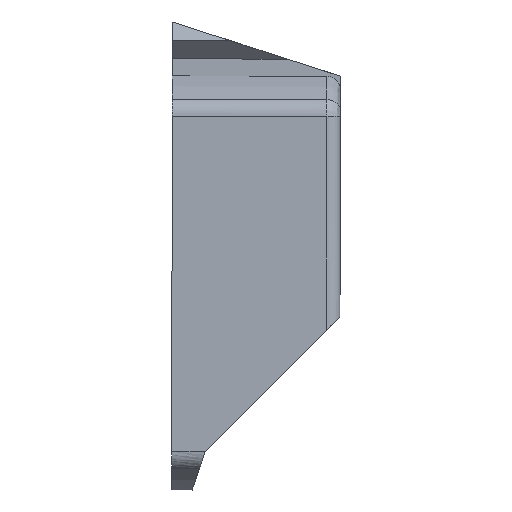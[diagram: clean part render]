
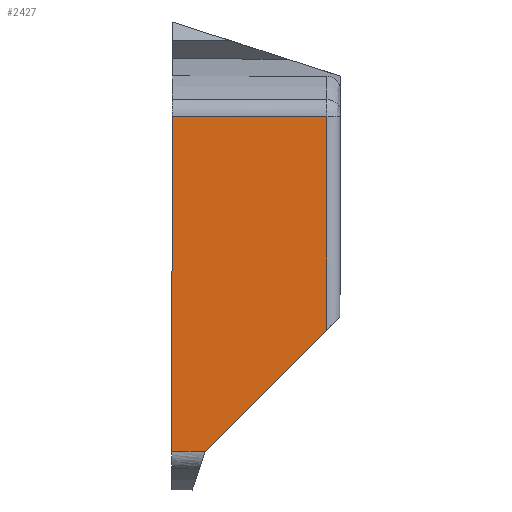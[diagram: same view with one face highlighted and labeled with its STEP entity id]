
A CAD part, front view. The second image highlights one B-rep face of the part: STEP entity #2427.
In plain terms, the highlighted planar face has unit normal (0, -1, 0).
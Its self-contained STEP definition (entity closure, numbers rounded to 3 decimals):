
#143=PLANE('',#2512);
#271=FACE_OUTER_BOUND('',#417,.T.);
#417=EDGE_LOOP('',(#2188,#2189,#2190,#2191,#2192,#2193));
#497=LINE('',#4180,#661);
#512=LINE('',#4357,#676);
#544=LINE('',#4589,#708);
#556=LINE('',#4790,#720);
#582=LINE('',#4938,#746);
#583=LINE('',#4939,#747);
#661=VECTOR('',#2600,10.);
#676=VECTOR('',#2637,10.);
#708=VECTOR('',#2695,10.);
#720=VECTOR('',#2737,10.);
#746=VECTOR('',#2803,10.);
#747=VECTOR('',#2804,10.);
#1038=VERTEX_POINT('',#4176);
#1040=VERTEX_POINT('',#4179);
#1071=VERTEX_POINT('',#4354);
#1072=VERTEX_POINT('',#4356);
#1112=VERTEX_POINT('',#4578);
#1133=VERTEX_POINT('',#4937);
#1351=EDGE_CURVE('',#1040,#1038,#497,.T.);
#1387=EDGE_CURVE('',#1071,#1072,#512,.T.);
#1437=EDGE_CURVE('',#1112,#1038,#544,.T.);
#1460=EDGE_CURVE('',#1072,#1112,#556,.T.);
#1491=EDGE_CURVE('',#1133,#1040,#582,.T.);
#1492=EDGE_CURVE('',#1071,#1133,#583,.T.);
#2188=ORIENTED_EDGE('',*,*,#1491,.T.);
#2189=ORIENTED_EDGE('',*,*,#1351,.T.);
#2190=ORIENTED_EDGE('',*,*,#1437,.F.);
#2191=ORIENTED_EDGE('',*,*,#1460,.F.);
#2192=ORIENTED_EDGE('',*,*,#1387,.F.);
#2193=ORIENTED_EDGE('',*,*,#1492,.T.);
#2427=ADVANCED_FACE('',(#271),#143,.T.);
#2512=AXIS2_PLACEMENT_3D('',#4936,#2801,#2802);
#2600=DIRECTION('',(0.707,0.,0.707));
#2637=DIRECTION('',(0.002,0.,1.));
#2695=DIRECTION('',(-0.002,0.,-1.));
#2737=DIRECTION('',(1.,0.,-0.002));
#2801=DIRECTION('center_axis',(0.,-1.,
0.));
#2802=DIRECTION('ref_axis',(0.,0.,-1.));
#2803=DIRECTION('',(1.,0.,-0.002));
#2804=DIRECTION('',(1.,0.,-0.002));
#4176=CARTESIAN_POINT('',(3065.21,309.834,87.299));
#4179=CARTESIAN_POINT('',(3047.186,309.834,69.275));
#4180=CARTESIAN_POINT('',(3069.38,309.834,91.469));
#4354=CARTESIAN_POINT('',(3042.178,309.834,69.283));
#4356=CARTESIAN_POINT('',(3042.265,309.834,119.164));
#4357=CARTESIAN_POINT('',(3042.259,309.834,115.43));
#4578=CARTESIAN_POINT('',(3065.265,309.834,119.124));
#4589=CARTESIAN_POINT('',(3065.237,309.834,102.824));
#4790=CARTESIAN_POINT('',(3047.265,309.834,119.156));
#4936=CARTESIAN_POINT('Origin',(3042.196,309.834,79.563));
#4937=CARTESIAN_POINT('',(3047.178,309.834,69.275));
#4938=CARTESIAN_POINT('',(3047.178,309.834,69.275));
#4939=CARTESIAN_POINT('',(3047.178,309.834,69.275));
